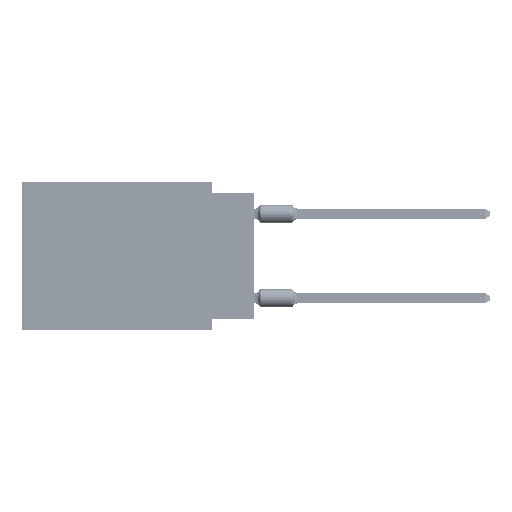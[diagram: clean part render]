
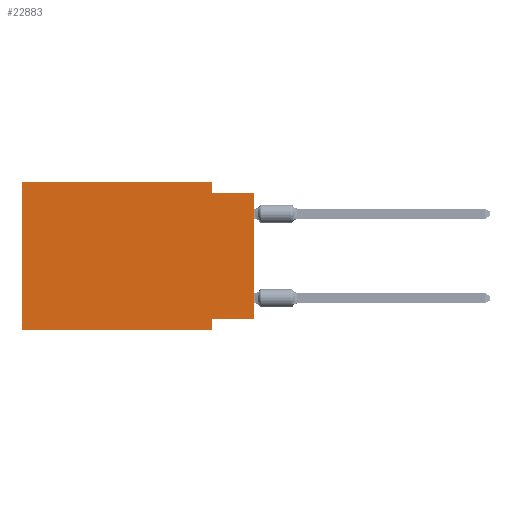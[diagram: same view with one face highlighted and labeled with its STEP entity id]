
A CAD part, left-side view. The second image highlights one B-rep face of the part: STEP entity #22883.
In plain terms, the highlighted planar face has unit normal (-1, 0, 0).
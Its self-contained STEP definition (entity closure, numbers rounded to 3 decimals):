
#2562 = CARTESIAN_POINT ( 'NONE',  ( 0., 13.97, 0. ) ) ;
#3094 = VECTOR ( 'NONE', #45919, 1000. ) ;
#4918 = ORIENTED_EDGE ( 'NONE', *, *, #54382, .F. ) ;
#4961 = VERTEX_POINT ( 'NONE', #63719 ) ;
#5094 = LINE ( 'NONE', #26898, #15305 ) ;
#5244 = CARTESIAN_POINT ( 'NONE',  ( 0., 0., -0.635 ) ) ;
#7945 = EDGE_CURVE ( 'NONE', #9871, #56884, #28366, .T. ) ;
#8046 = CARTESIAN_POINT ( 'NONE',  ( 0., 2.54, -8.89 ) ) ;
#9458 = VERTEX_POINT ( 'NONE', #16159 ) ;
#9871 = VERTEX_POINT ( 'NONE', #35172 ) ;
#11565 = ORIENTED_EDGE ( 'NONE', *, *, #7945, .F. ) ;
#12393 = CARTESIAN_POINT ( 'NONE',  ( 0., 2.54, -0.635 ) ) ;
#12397 = ORIENTED_EDGE ( 'NONE', *, *, #38773, .T. ) ;
#15305 = VECTOR ( 'NONE', #70528, 1000. ) ;
#15824 = CARTESIAN_POINT ( 'NONE',  ( 0., 2.54, 0. ) ) ;
#16023 = LINE ( 'NONE', #42117, #28316 ) ;
#16159 = CARTESIAN_POINT ( 'NONE',  ( 0., 0., -0.635 ) ) ;
#17959 = EDGE_CURVE ( 'NONE', #56884, #58181, #5094, .T. ) ;
#18791 = DIRECTION ( 'NONE',  ( 0., 0., -1. ) ) ;
#18939 = VECTOR ( 'NONE', #42785, 1000. ) ;
#20643 = EDGE_CURVE ( 'NONE', #27679, #4961, #45568, .T. ) ;
#22883 = ADVANCED_FACE ( 'NONE', ( #51540 ), #39121, .F. ) ;
#23705 = AXIS2_PLACEMENT_3D ( 'NONE', #2562, #56537, #46522 ) ;
#25775 = VECTOR ( 'NONE', #18791, 1000. ) ;
#26898 = CARTESIAN_POINT ( 'NONE',  ( 0., 13.97, 0. ) ) ;
#27679 = VERTEX_POINT ( 'NONE', #29392 ) ;
#28316 = VECTOR ( 'NONE', #69989, 1000. ) ;
#28366 = LINE ( 'NONE', #61949, #44555 ) ;
#29392 = CARTESIAN_POINT ( 'NONE',  ( 0., 2.54, -8.255 ) ) ;
#33757 = LINE ( 'NONE', #60251, #53260 ) ;
#34066 = DIRECTION ( 'NONE',  ( 0., 0., 1. ) ) ;
#35172 = CARTESIAN_POINT ( 'NONE',  ( 0., 13.97, -8.89 ) ) ;
#35779 = ORIENTED_EDGE ( 'NONE', *, *, #52696, .F. ) ;
#36268 = CARTESIAN_POINT ( 'NONE',  ( 0., 2.54, 0. ) ) ;
#38773 = EDGE_CURVE ( 'NONE', #53351, #9458, #44856, .T. ) ;
#39121 = PLANE ( 'NONE',  #23705 ) ;
#40919 = DIRECTION ( 'NONE',  ( 0., 0., 1. ) ) ;
#41992 = LINE ( 'NONE', #36268, #25775 ) ;
#42117 = CARTESIAN_POINT ( 'NONE',  ( 0., 13.97, -8.89 ) ) ;
#42785 = DIRECTION ( 'NONE',  ( 0., -1., 0. ) ) ;
#43313 = EDGE_CURVE ( 'NONE', #9871, #4961, #16023, .T. ) ;
#44555 = VECTOR ( 'NONE', #34066, 1000. ) ;
#44845 = DIRECTION ( 'NONE',  ( 0., 1., 0. ) ) ;
#44856 = LINE ( 'NONE', #56645, #65139 ) ;
#45568 = LINE ( 'NONE', #8046, #3094 ) ;
#45919 = DIRECTION ( 'NONE',  ( 0., 0., -1. ) ) ;
#46522 = DIRECTION ( 'NONE',  ( 0., 0., -1. ) ) ;
#49238 = EDGE_CURVE ( 'NONE', #59049, #9458, #65304, .T. ) ;
#51241 = ORIENTED_EDGE ( 'NONE', *, *, #43313, .T. ) ;
#51540 = FACE_OUTER_BOUND ( 'NONE', #57403, .T. ) ;
#52696 = EDGE_CURVE ( 'NONE', #53351, #27679, #33757, .T. ) ;
#53260 = VECTOR ( 'NONE', #44845, 1000. ) ;
#53351 = VERTEX_POINT ( 'NONE', #66518 ) ;
#54382 = EDGE_CURVE ( 'NONE', #58181, #59049, #41992, .T. ) ;
#56537 = DIRECTION ( 'NONE',  ( 1., 0., 0. ) ) ;
#56645 = CARTESIAN_POINT ( 'NONE',  ( 0., 0., 0. ) ) ;
#56884 = VERTEX_POINT ( 'NONE', #68838 ) ;
#57403 = EDGE_LOOP ( 'NONE', ( #12397, #57971, #4918, #67160, #11565, #51241, #68182, #35779 ) ) ;
#57971 = ORIENTED_EDGE ( 'NONE', *, *, #49238, .F. ) ;
#58181 = VERTEX_POINT ( 'NONE', #15824 ) ;
#59049 = VERTEX_POINT ( 'NONE', #12393 ) ;
#60251 = CARTESIAN_POINT ( 'NONE',  ( 0., 0., -8.255 ) ) ;
#61949 = CARTESIAN_POINT ( 'NONE',  ( 0., 13.97, 0. ) ) ;
#63719 = CARTESIAN_POINT ( 'NONE',  ( 0., 2.54, -8.89 ) ) ;
#65139 = VECTOR ( 'NONE', #40919, 1000. ) ;
#65304 = LINE ( 'NONE', #5244, #18939 ) ;
#66518 = CARTESIAN_POINT ( 'NONE',  ( 0., 0., -8.255 ) ) ;
#67160 = ORIENTED_EDGE ( 'NONE', *, *, #17959, .F. ) ;
#68182 = ORIENTED_EDGE ( 'NONE', *, *, #20643, .F. ) ;
#68838 = CARTESIAN_POINT ( 'NONE',  ( 0., 13.97, 0. ) ) ;
#69989 = DIRECTION ( 'NONE',  ( 0., -1., 0. ) ) ;
#70528 = DIRECTION ( 'NONE',  ( 0., -1., 0. ) ) ;
